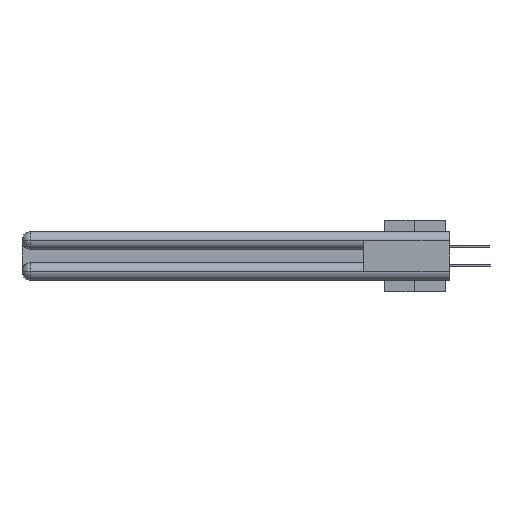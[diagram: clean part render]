
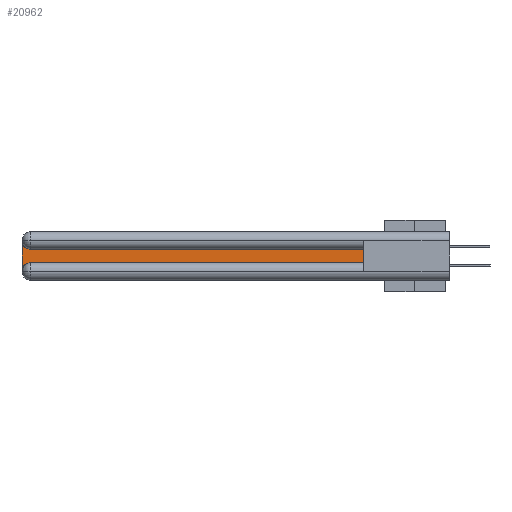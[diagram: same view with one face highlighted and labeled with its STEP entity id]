
A CAD part, left-side view. The second image highlights one B-rep face of the part: STEP entity #20962.
In plain terms, the highlighted planar face has unit normal (-1, 0, 0).
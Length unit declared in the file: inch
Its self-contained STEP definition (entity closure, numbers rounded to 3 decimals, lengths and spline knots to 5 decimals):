
#974 = VERTEX_POINT ( 'NONE', #2371 ) ;
#1530 = CARTESIAN_POINT ( 'NONE',  ( 0.075, 2.94, -0.1225 ) ) ;
#2371 = CARTESIAN_POINT ( 'NONE',  ( 0.075, 0.6, -0.2175 ) ) ;
#4625 = DIRECTION ( 'NONE',  ( 0., 0., -1. ) ) ;
#4847 = AXIS2_PLACEMENT_3D ( 'NONE', #13328, #36324, #6027 ) ;
#5084 = FACE_OUTER_BOUND ( 'NONE', #12029, .T. ) ;
#5292 = AXIS2_PLACEMENT_3D ( 'NONE', #14449, #35573, #15509 ) ;
#6027 = DIRECTION ( 'NONE',  ( 0., 0., -1. ) ) ;
#8899 = ORIENTED_EDGE ( 'NONE', *, *, #19568, .T. ) ;
#8926 = CARTESIAN_POINT ( 'NONE',  ( 0.075, 0.6, -0.2175 ) ) ;
#9049 = LINE ( 'NONE', #15665, #18941 ) ;
#10786 = EDGE_CURVE ( 'NONE', #34332, #43168, #41497, .T. ) ;
#11099 = EDGE_CURVE ( 'NONE', #19954, #23686, #9049, .T. ) ;
#12029 = EDGE_LOOP ( 'NONE', ( #22299, #8899, #41236, #15061, #27563, #16859 ) ) ;
#13328 = CARTESIAN_POINT ( 'NONE',  ( 0.075, 2.94, -0.2775 ) ) ;
#14449 = CARTESIAN_POINT ( 'NONE',  ( 0.075, 2.94, -0.0625 ) ) ;
#15061 = ORIENTED_EDGE ( 'NONE', *, *, #17363, .T. ) ;
#15509 = DIRECTION ( 'NONE',  ( 0., 0., -1. ) ) ;
#15665 = CARTESIAN_POINT ( 'NONE',  ( 0.075, 0.6, -0.1225 ) ) ;
#16859 = ORIENTED_EDGE ( 'NONE', *, *, #18617, .T. ) ;
#17363 = EDGE_CURVE ( 'NONE', #43168, #35075, #34031, .T. ) ;
#17548 = CARTESIAN_POINT ( 'NONE',  ( 0.075, 0.6, -0.2175 ) ) ;
#17904 = PLANE ( 'NONE',  #19776 ) ;
#18617 = EDGE_CURVE ( 'NONE', #974, #19954, #21426, .T. ) ;
#18941 = VECTOR ( 'NONE', #23167, 39.37008 ) ;
#19568 = EDGE_CURVE ( 'NONE', #23686, #34332, #32438, .T. ) ;
#19776 = AXIS2_PLACEMENT_3D ( 'NONE', #24522, #24676, #4625 ) ;
#19954 = VERTEX_POINT ( 'NONE', #34019 ) ;
#20594 = CARTESIAN_POINT ( 'NONE',  ( 0.075, 3., -0.2775 ) ) ;
#20886 = VECTOR ( 'NONE', #25330, 39.37008 ) ;
#20962 = ADVANCED_FACE ( 'NONE', ( #5084 ), #17904, .F. ) ;
#21426 = LINE ( 'NONE', #8926, #20886 ) ;
#22299 = ORIENTED_EDGE ( 'NONE', *, *, #11099, .T. ) ;
#22638 = VECTOR ( 'NONE', #25337, 39.37008 ) ;
#23167 = DIRECTION ( 'NONE',  ( 0., 1., 0. ) ) ;
#23686 = VERTEX_POINT ( 'NONE', #1530 ) ;
#24522 = CARTESIAN_POINT ( 'NONE',  ( 0.075, 3., -0.1225 ) ) ;
#24676 = DIRECTION ( 'NONE',  ( 1., 0., 0. ) ) ;
#24899 = EDGE_CURVE ( 'NONE', #35075, #974, #29943, .T. ) ;
#25330 = DIRECTION ( 'NONE',  ( 0., 0., 1. ) ) ;
#25337 = DIRECTION ( 'NONE',  ( 0., -1., 0. ) ) ;
#25879 = CARTESIAN_POINT ( 'NONE',  ( 0.075, 3., -0.2175 ) ) ;
#27563 = ORIENTED_EDGE ( 'NONE', *, *, #24899, .T. ) ;
#29943 = LINE ( 'NONE', #17548, #22638 ) ;
#32438 = CIRCLE ( 'NONE', #5292, 0.06 ) ;
#32617 = VECTOR ( 'NONE', #39435, 39.37008 ) ;
#33529 = CARTESIAN_POINT ( 'NONE',  ( 0.075, 3., -0.0625 ) ) ;
#34019 = CARTESIAN_POINT ( 'NONE',  ( 0.075, 0.6, -0.1225 ) ) ;
#34031 = CIRCLE ( 'NONE', #4847, 0.06 ) ;
#34332 = VERTEX_POINT ( 'NONE', #33529 ) ;
#34658 = CARTESIAN_POINT ( 'NONE',  ( 0.075, 2.94, -0.2175 ) ) ;
#35075 = VERTEX_POINT ( 'NONE', #34658 ) ;
#35573 = DIRECTION ( 'NONE',  ( 1., 0., 0. ) ) ;
#36324 = DIRECTION ( 'NONE',  ( 1., 0., 0. ) ) ;
#39435 = DIRECTION ( 'NONE',  ( 0., 0., -1. ) ) ;
#41236 = ORIENTED_EDGE ( 'NONE', *, *, #10786, .T. ) ;
#41497 = LINE ( 'NONE', #25879, #32617 ) ;
#43168 = VERTEX_POINT ( 'NONE', #20594 ) ;
